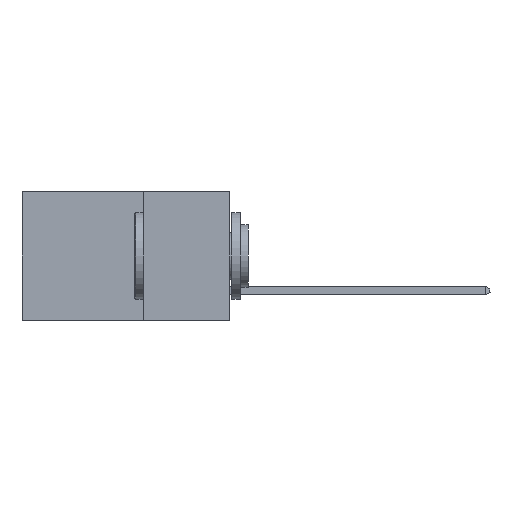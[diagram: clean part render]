
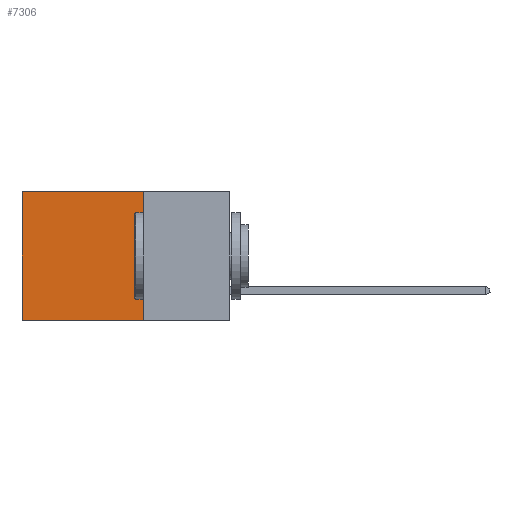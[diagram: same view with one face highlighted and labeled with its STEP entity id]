
A CAD part, left-side view. The second image highlights one B-rep face of the part: STEP entity #7306.
In plain terms, the highlighted planar face has unit normal (-1, 0, 0).
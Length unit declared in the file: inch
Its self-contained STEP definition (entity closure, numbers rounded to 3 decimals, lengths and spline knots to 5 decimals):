
#614 = DIRECTION ( 'NONE',  ( 0., 1., 0. ) ) ;
#1383 = VERTEX_POINT ( 'NONE', #16729 ) ;
#2978 = EDGE_LOOP ( 'NONE', ( #14446, #19939, #15927, #6576 ) ) ;
#4157 = LINE ( 'NONE', #21236, #14291 ) ;
#4915 = LINE ( 'NONE', #28413, #19407 ) ;
#5867 = CARTESIAN_POINT ( 'NONE',  ( 0.298, 0.6, 0. ) ) ;
#6576 = ORIENTED_EDGE ( 'NONE', *, *, #23790, .T. ) ;
#6599 = DIRECTION ( 'NONE',  ( 0., 0., -1. ) ) ;
#6794 = CARTESIAN_POINT ( 'NONE',  ( 0.298, 0.25, 0. ) ) ;
#7306 = ADVANCED_FACE ( 'NONE', ( #13031 ), #15944, .F. ) ;
#7328 = EDGE_CURVE ( 'NONE', #29847, #1383, #27591, .T. ) ;
#9105 = CARTESIAN_POINT ( 'NONE',  ( 0.298, 0.25, 0. ) ) ;
#9378 = VECTOR ( 'NONE', #11455, 39.37008 ) ;
#9557 = DIRECTION ( 'NONE',  ( 0., 1., 0. ) ) ;
#11455 = DIRECTION ( 'NONE',  ( 0., 0., -1. ) ) ;
#13031 = FACE_OUTER_BOUND ( 'NONE', #2978, .T. ) ;
#14291 = VECTOR ( 'NONE', #9557, 39.37008 ) ;
#14446 = ORIENTED_EDGE ( 'NONE', *, *, #23353, .T. ) ;
#15927 = ORIENTED_EDGE ( 'NONE', *, *, #7328, .F. ) ;
#15944 = PLANE ( 'NONE',  #29824 ) ;
#16729 = CARTESIAN_POINT ( 'NONE',  ( 0.298, 0.25, -0.37 ) ) ;
#19407 = VECTOR ( 'NONE', #614, 39.37008 ) ;
#19939 = ORIENTED_EDGE ( 'NONE', *, *, #23286, .F. ) ;
#21236 = CARTESIAN_POINT ( 'NONE',  ( 0.298, 0.25, 0. ) ) ;
#21270 = CARTESIAN_POINT ( 'NONE',  ( 0.298, 0.6, -0.37 ) ) ;
#21581 = LINE ( 'NONE', #28905, #28880 ) ;
#23140 = VERTEX_POINT ( 'NONE', #21270 ) ;
#23286 = EDGE_CURVE ( 'NONE', #1383, #23140, #4915, .T. ) ;
#23353 = EDGE_CURVE ( 'NONE', #27521, #23140, #21581, .T. ) ;
#23790 = EDGE_CURVE ( 'NONE', #29847, #27521, #4157, .T. ) ;
#25137 = DIRECTION ( 'NONE',  ( 1., 0., 0. ) ) ;
#26870 = DIRECTION ( 'NONE',  ( 0., 0., -1. ) ) ;
#27521 = VERTEX_POINT ( 'NONE', #5867 ) ;
#27591 = LINE ( 'NONE', #9105, #9378 ) ;
#28413 = CARTESIAN_POINT ( 'NONE',  ( 0.298, 0.25, -0.37 ) ) ;
#28880 = VECTOR ( 'NONE', #26870, 39.37008 ) ;
#28905 = CARTESIAN_POINT ( 'NONE',  ( 0.298, 0.6, 0. ) ) ;
#29434 = CARTESIAN_POINT ( 'NONE',  ( 0.298, 0.25, 0. ) ) ;
#29824 = AXIS2_PLACEMENT_3D ( 'NONE', #6794, #25137, #6599 ) ;
#29847 = VERTEX_POINT ( 'NONE', #29434 ) ;
